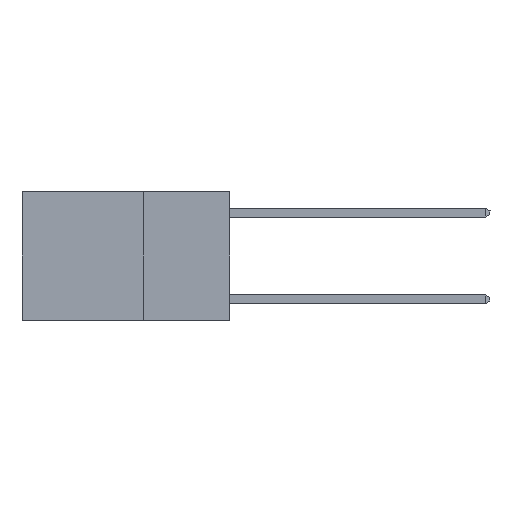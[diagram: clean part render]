
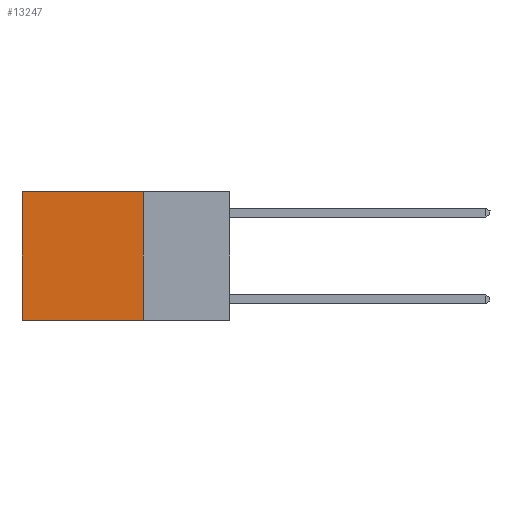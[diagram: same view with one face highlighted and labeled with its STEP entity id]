
A CAD part, left-side view. The second image highlights one B-rep face of the part: STEP entity #13247.
In plain terms, the highlighted planar face has unit normal (-1, 0, 0).
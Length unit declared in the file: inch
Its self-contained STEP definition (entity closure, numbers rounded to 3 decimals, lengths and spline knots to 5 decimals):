
#392 = CARTESIAN_POINT ( 'NONE',  ( 0.2625, 0.25, 0. ) ) ;
#782 = VERTEX_POINT ( 'NONE', #6035 ) ;
#1489 = EDGE_CURVE ( 'NONE', #9249, #11987, #10199, .T. ) ;
#1687 = DIRECTION ( 'NONE',  ( 0., 0., -1. ) ) ;
#1754 = VERTEX_POINT ( 'NONE', #5078 ) ;
#2249 = EDGE_LOOP ( 'NONE', ( #5680, #7169, #10338, #13475 ) ) ;
#5078 = CARTESIAN_POINT ( 'NONE',  ( 0.2625, 0.25, 0. ) ) ;
#5680 = ORIENTED_EDGE ( 'NONE', *, *, #1489, .T. ) ;
#5777 = FACE_OUTER_BOUND ( 'NONE', #2249, .T. ) ;
#6035 = CARTESIAN_POINT ( 'NONE',  ( 0.2625, 0.25, -0.37 ) ) ;
#6330 = VECTOR ( 'NONE', #13734, 39.37008 ) ;
#6349 = EDGE_CURVE ( 'NONE', #1754, #9249, #12647, .T. ) ;
#6683 = CARTESIAN_POINT ( 'NONE',  ( 0.2625, 0.25, 0. ) ) ;
#7169 = ORIENTED_EDGE ( 'NONE', *, *, #14839, .F. ) ;
#7210 = VECTOR ( 'NONE', #9218, 39.37008 ) ;
#8042 = CARTESIAN_POINT ( 'NONE',  ( 0.2625, 0.25, 0. ) ) ;
#8250 = CARTESIAN_POINT ( 'NONE',  ( 0.2625, 0.25, -0.37 ) ) ;
#8439 = EDGE_CURVE ( 'NONE', #1754, #782, #9990, .T. ) ;
#8572 = AXIS2_PLACEMENT_3D ( 'NONE', #392, #8949, #1687 ) ;
#8949 = DIRECTION ( 'NONE',  ( 1., 0., 0. ) ) ;
#9218 = DIRECTION ( 'NONE',  ( 0., 0., -1. ) ) ;
#9249 = VERTEX_POINT ( 'NONE', #14014 ) ;
#9252 = DIRECTION ( 'NONE',  ( 0., 0., -1. ) ) ;
#9264 = CARTESIAN_POINT ( 'NONE',  ( 0.2625, 0.6, 0. ) ) ;
#9437 = DIRECTION ( 'NONE',  ( 0., 1., 0. ) ) ;
#9812 = VECTOR ( 'NONE', #9252, 39.37008 ) ;
#9990 = LINE ( 'NONE', #8042, #7210 ) ;
#9998 = VECTOR ( 'NONE', #9437, 39.37008 ) ;
#10090 = CARTESIAN_POINT ( 'NONE',  ( 0.2625, 0.6, -0.37 ) ) ;
#10199 = LINE ( 'NONE', #9264, #9812 ) ;
#10338 = ORIENTED_EDGE ( 'NONE', *, *, #8439, .F. ) ;
#10370 = LINE ( 'NONE', #8250, #9998 ) ;
#11987 = VERTEX_POINT ( 'NONE', #10090 ) ;
#12502 = PLANE ( 'NONE',  #8572 ) ;
#12647 = LINE ( 'NONE', #6683, #6330 ) ;
#13247 = ADVANCED_FACE ( 'NONE', ( #5777 ), #12502, .F. ) ;
#13475 = ORIENTED_EDGE ( 'NONE', *, *, #6349, .T. ) ;
#13734 = DIRECTION ( 'NONE',  ( 0., 1., 0. ) ) ;
#14014 = CARTESIAN_POINT ( 'NONE',  ( 0.2625, 0.6, 0. ) ) ;
#14839 = EDGE_CURVE ( 'NONE', #782, #11987, #10370, .T. ) ;
